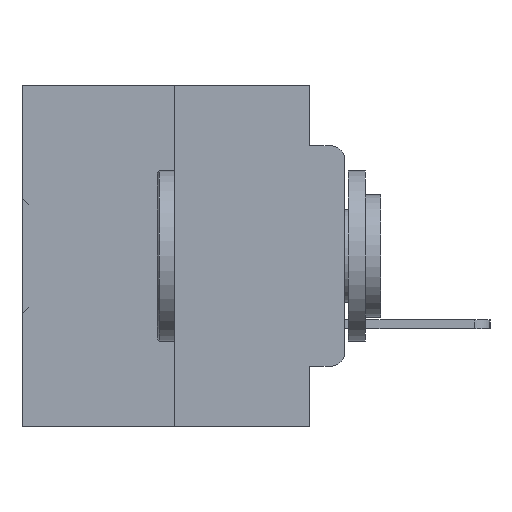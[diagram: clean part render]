
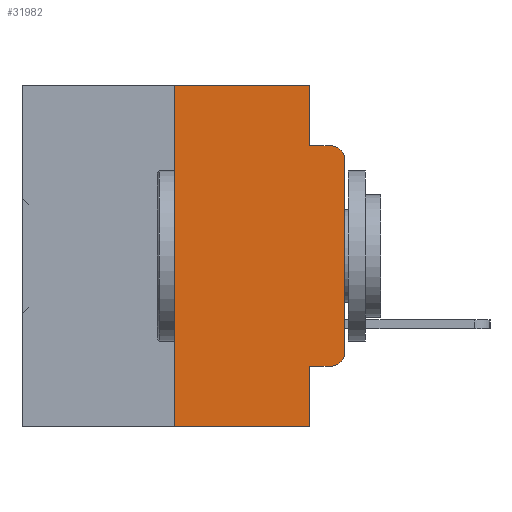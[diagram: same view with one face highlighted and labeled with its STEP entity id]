
A CAD part, left-side view. The second image highlights one B-rep face of the part: STEP entity #31982.
In plain terms, the highlighted planar face has unit normal (-1, 0, 0).
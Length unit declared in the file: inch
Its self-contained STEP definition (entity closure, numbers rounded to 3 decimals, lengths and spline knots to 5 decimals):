
#368 = VERTEX_POINT ( 'NONE', #34636 ) ;
#958 = CARTESIAN_POINT ( 'NONE',  ( 0., 0.051, -0.4115 ) ) ;
#1068 = VERTEX_POINT ( 'NONE', #958 ) ;
#1075 = EDGE_CURVE ( 'NONE', #14727, #15137, #32343, .T. ) ;
#1520 = LINE ( 'NONE', #22496, #16301 ) ;
#1556 = VECTOR ( 'NONE', #15041, 39.37008 ) ;
#1829 = DIRECTION ( 'NONE',  ( 0., -1., 0. ) ) ;
#2037 = EDGE_CURVE ( 'NONE', #15137, #7716, #10874, .T. ) ;
#2765 = VECTOR ( 'NONE', #8872, 39.37008 ) ;
#3238 = EDGE_CURVE ( 'NONE', #5842, #368, #4577, .T. ) ;
#3695 = CARTESIAN_POINT ( 'NONE',  ( 0., 0.02, -0.3915 ) ) ;
#4018 = ORIENTED_EDGE ( 'NONE', *, *, #6235, .T. ) ;
#4577 = CIRCLE ( 'NONE', #16733, 0.02 ) ;
#4851 = ORIENTED_EDGE ( 'NONE', *, *, #2037, .F. ) ;
#5317 = VECTOR ( 'NONE', #1829, 39.37008 ) ;
#5842 = VERTEX_POINT ( 'NONE', #27154 ) ;
#6091 = PLANE ( 'NONE',  #28721 ) ;
#6235 = EDGE_CURVE ( 'NONE', #1068, #5842, #27799, .T. ) ;
#6936 = DIRECTION ( 'NONE',  ( 0., 0., -1. ) ) ;
#7303 = ORIENTED_EDGE ( 'NONE', *, *, #28293, .T. ) ;
#7423 = ORIENTED_EDGE ( 'NONE', *, *, #15216, .F. ) ;
#7468 = DIRECTION ( 'NONE',  ( 0., -1., 0. ) ) ;
#7615 = EDGE_CURVE ( 'NONE', #1068, #14140, #8951, .T. ) ;
#7716 = VERTEX_POINT ( 'NONE', #34784 ) ;
#8218 = CARTESIAN_POINT ( 'NONE',  ( 0., 0.051, -0.4115 ) ) ;
#8872 = DIRECTION ( 'NONE',  ( 0., -1., 0. ) ) ;
#8951 = LINE ( 'NONE', #31479, #1556 ) ;
#9224 = ORIENTED_EDGE ( 'NONE', *, *, #23520, .T. ) ;
#9392 = CARTESIAN_POINT ( 'NONE',  ( 0., 0.25, 0. ) ) ;
#9415 = ORIENTED_EDGE ( 'NONE', *, *, #7615, .F. ) ;
#10385 = VECTOR ( 'NONE', #7468, 39.37008 ) ;
#10440 = CIRCLE ( 'NONE', #16365, 0.02 ) ;
#10874 = LINE ( 'NONE', #30942, #32821 ) ;
#11064 = DIRECTION ( 'NONE',  ( -1., 0., 0. ) ) ;
#11278 = CARTESIAN_POINT ( 'NONE',  ( 0., 0.25, 0. ) ) ;
#12291 = VERTEX_POINT ( 'NONE', #13926 ) ;
#12656 = CARTESIAN_POINT ( 'NONE',  ( 0., 0.051, -0.5 ) ) ;
#13029 = VECTOR ( 'NONE', #29383, 39.37008 ) ;
#13926 = CARTESIAN_POINT ( 'NONE',  ( 0., 0., -0.1085 ) ) ;
#14140 = VERTEX_POINT ( 'NONE', #12656 ) ;
#14491 = DIRECTION ( 'NONE',  ( 0., 0., -1. ) ) ;
#14727 = VERTEX_POINT ( 'NONE', #9392 ) ;
#14907 = CARTESIAN_POINT ( 'NONE',  ( 0., 0.473, 0. ) ) ;
#14952 = ORIENTED_EDGE ( 'NONE', *, *, #1075, .F. ) ;
#15041 = DIRECTION ( 'NONE',  ( 0., 0., -1. ) ) ;
#15137 = VERTEX_POINT ( 'NONE', #22044 ) ;
#15216 = EDGE_CURVE ( 'NONE', #25741, #14727, #21026, .T. ) ;
#16301 = VECTOR ( 'NONE', #25279, 39.37008 ) ;
#16365 = AXIS2_PLACEMENT_3D ( 'NONE', #27606, #11064, #30340 ) ;
#16733 = AXIS2_PLACEMENT_3D ( 'NONE', #3695, #23724, #6936 ) ;
#17679 = DIRECTION ( 'NONE',  ( 1., 0., 0. ) ) ;
#19871 = EDGE_LOOP ( 'NONE', ( #7303, #9224, #31223, #4851, #14952, #7423, #26222, #9415, #4018, #26703 ) ) ;
#20258 = FACE_OUTER_BOUND ( 'NONE', #19871, .T. ) ;
#21026 = LINE ( 'NONE', #11278, #26620 ) ;
#22044 = CARTESIAN_POINT ( 'NONE',  ( 0., 0.051, 0. ) ) ;
#22496 = CARTESIAN_POINT ( 'NONE',  ( 0., 0.473, -0.5 ) ) ;
#23520 = EDGE_CURVE ( 'NONE', #12291, #35946, #10440, .T. ) ;
#23724 = DIRECTION ( 'NONE',  ( -1., 0., 0. ) ) ;
#24100 = CARTESIAN_POINT ( 'NONE',  ( 0., 0.02, -0.0885 ) ) ;
#24664 = EDGE_CURVE ( 'NONE', #7716, #35946, #33713, .T. ) ;
#25279 = DIRECTION ( 'NONE',  ( 0., -1., 0. ) ) ;
#25457 = CARTESIAN_POINT ( 'NONE',  ( 0., 0.051, -0.0885 ) ) ;
#25741 = VERTEX_POINT ( 'NONE', #26244 ) ;
#26222 = ORIENTED_EDGE ( 'NONE', *, *, #36192, .T. ) ;
#26244 = CARTESIAN_POINT ( 'NONE',  ( 0., 0.25, -0.5 ) ) ;
#26620 = VECTOR ( 'NONE', #33273, 39.37008 ) ;
#26653 = CARTESIAN_POINT ( 'NONE',  ( 0., 0., 0. ) ) ;
#26703 = ORIENTED_EDGE ( 'NONE', *, *, #3238, .T. ) ;
#27154 = CARTESIAN_POINT ( 'NONE',  ( 0., 0.02, -0.4115 ) ) ;
#27606 = CARTESIAN_POINT ( 'NONE',  ( 0., 0.02, -0.1085 ) ) ;
#27799 = LINE ( 'NONE', #8218, #5317 ) ;
#28293 = EDGE_CURVE ( 'NONE', #368, #12291, #34936, .T. ) ;
#28721 = AXIS2_PLACEMENT_3D ( 'NONE', #14907, #17679, #36826 ) ;
#29383 = DIRECTION ( 'NONE',  ( 0., 0., 1. ) ) ;
#29699 = CARTESIAN_POINT ( 'NONE',  ( 0., 0.473, 0. ) ) ;
#30340 = DIRECTION ( 'NONE',  ( 0., 0., -1. ) ) ;
#30942 = CARTESIAN_POINT ( 'NONE',  ( 0., 0.051, 0. ) ) ;
#31223 = ORIENTED_EDGE ( 'NONE', *, *, #24664, .F. ) ;
#31479 = CARTESIAN_POINT ( 'NONE',  ( 0., 0.051, 0. ) ) ;
#31982 = ADVANCED_FACE ( 'NONE', ( #20258 ), #6091, .F. ) ;
#32343 = LINE ( 'NONE', #29699, #10385 ) ;
#32821 = VECTOR ( 'NONE', #14491, 39.37008 ) ;
#33273 = DIRECTION ( 'NONE',  ( 0., 0., 1. ) ) ;
#33713 = LINE ( 'NONE', #25457, #2765 ) ;
#34636 = CARTESIAN_POINT ( 'NONE',  ( 0., 0., -0.3915 ) ) ;
#34784 = CARTESIAN_POINT ( 'NONE',  ( 0., 0.051, -0.0885 ) ) ;
#34936 = LINE ( 'NONE', #26653, #13029 ) ;
#35946 = VERTEX_POINT ( 'NONE', #24100 ) ;
#36192 = EDGE_CURVE ( 'NONE', #25741, #14140, #1520, .T. ) ;
#36826 = DIRECTION ( 'NONE',  ( 0., 0., -1. ) ) ;
